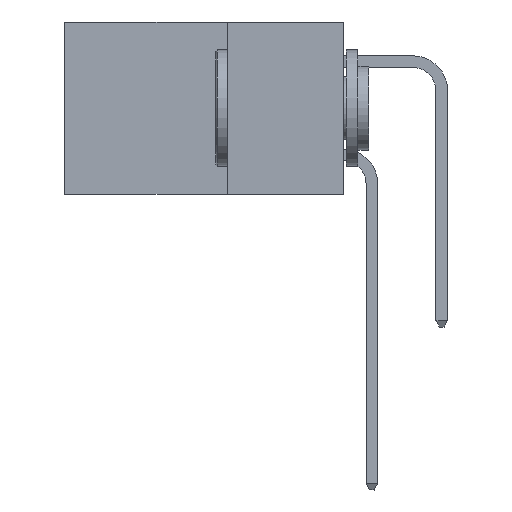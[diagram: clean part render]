
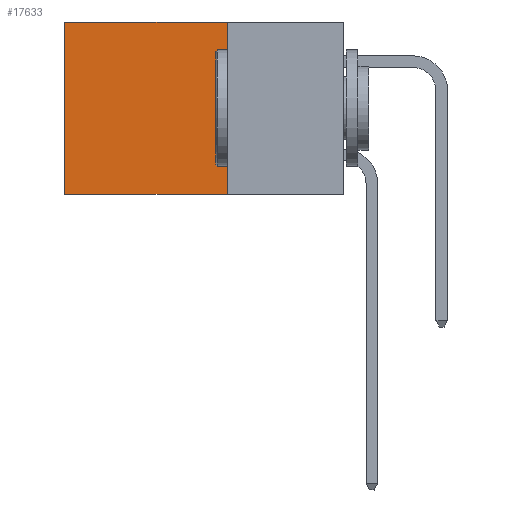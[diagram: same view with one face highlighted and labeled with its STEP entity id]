
A CAD part, left-side view. The second image highlights one B-rep face of the part: STEP entity #17633.
In plain terms, the highlighted planar face has unit normal (-1, 0, 0).
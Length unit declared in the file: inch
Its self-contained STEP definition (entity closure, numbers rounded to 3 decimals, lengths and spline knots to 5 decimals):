
#902 = FACE_OUTER_BOUND ( 'NONE', #10530, .T. ) ;
#2066 = ORIENTED_EDGE ( 'NONE', *, *, #4750, .F. ) ;
#3909 = DIRECTION ( 'NONE',  ( 0., 1., 0. ) ) ;
#4638 = CARTESIAN_POINT ( 'NONE',  ( 0.2615, 0.6, 0. ) ) ;
#4750 = EDGE_CURVE ( 'NONE', #5123, #19489, #15776, .T. ) ;
#5123 = VERTEX_POINT ( 'NONE', #11577 ) ;
#5358 = CARTESIAN_POINT ( 'NONE',  ( 0.2615, 0.25, -0.37 ) ) ;
#5367 = VECTOR ( 'NONE', #3909, 39.37008 ) ;
#5757 = CARTESIAN_POINT ( 'NONE',  ( 0.2615, 0.6, -0.37 ) ) ;
#6077 = LINE ( 'NONE', #23666, #5367 ) ;
#10018 = VECTOR ( 'NONE', #19435, 39.37008 ) ;
#10072 = DIRECTION ( 'NONE',  ( 0., 1., 0. ) ) ;
#10530 = EDGE_LOOP ( 'NONE', ( #12346, #26680, #2066, #24522 ) ) ;
#11577 = CARTESIAN_POINT ( 'NONE',  ( 0.2615, 0.25, 0. ) ) ;
#12175 = DIRECTION ( 'NONE',  ( 0., 0., -1. ) ) ;
#12346 = ORIENTED_EDGE ( 'NONE', *, *, #25836, .T. ) ;
#12567 = EDGE_CURVE ( 'NONE', #19489, #18124, #23175, .T. ) ;
#13898 = PLANE ( 'NONE',  #22355 ) ;
#14185 = DIRECTION ( 'NONE',  ( 1., 0., 0. ) ) ;
#14572 = LINE ( 'NONE', #5757, #10018 ) ;
#15776 = LINE ( 'NONE', #27162, #25064 ) ;
#16678 = CARTESIAN_POINT ( 'NONE',  ( 0.2615, 0.25, -0.37 ) ) ;
#17633 = ADVANCED_FACE ( 'NONE', ( #902 ), #13898, .F. ) ;
#18124 = VERTEX_POINT ( 'NONE', #23768 ) ;
#18759 = VERTEX_POINT ( 'NONE', #4638 ) ;
#19435 = DIRECTION ( 'NONE',  ( 0., 0., -1. ) ) ;
#19489 = VERTEX_POINT ( 'NONE', #26252 ) ;
#20858 = VECTOR ( 'NONE', #10072, 39.37008 ) ;
#22355 = AXIS2_PLACEMENT_3D ( 'NONE', #5358, #14185, #22969 ) ;
#22969 = DIRECTION ( 'NONE',  ( 0., 0., -1. ) ) ;
#23175 = LINE ( 'NONE', #16678, #20858 ) ;
#23666 = CARTESIAN_POINT ( 'NONE',  ( 0.2615, 0.25, 0. ) ) ;
#23768 = CARTESIAN_POINT ( 'NONE',  ( 0.2615, 0.6, -0.37 ) ) ;
#24522 = ORIENTED_EDGE ( 'NONE', *, *, #25437, .T. ) ;
#25064 = VECTOR ( 'NONE', #12175, 39.37008 ) ;
#25437 = EDGE_CURVE ( 'NONE', #5123, #18759, #6077, .T. ) ;
#25836 = EDGE_CURVE ( 'NONE', #18759, #18124, #14572, .T. ) ;
#26252 = CARTESIAN_POINT ( 'NONE',  ( 0.2615, 0.25, -0.37 ) ) ;
#26680 = ORIENTED_EDGE ( 'NONE', *, *, #12567, .F. ) ;
#27162 = CARTESIAN_POINT ( 'NONE',  ( 0.2615, 0.25, -0.37 ) ) ;
